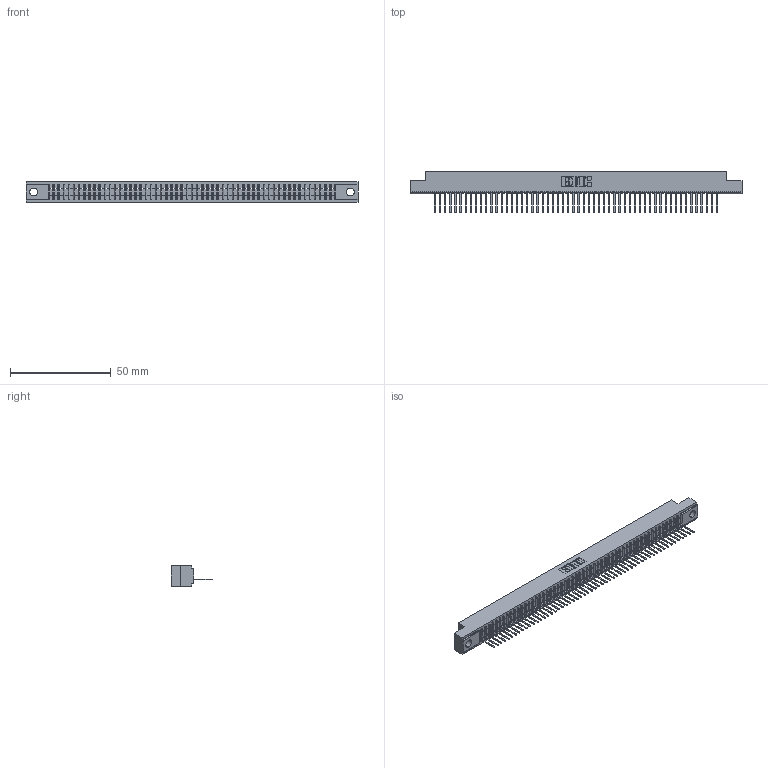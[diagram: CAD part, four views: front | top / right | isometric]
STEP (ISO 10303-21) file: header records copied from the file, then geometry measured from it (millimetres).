
FILE_DESCRIPTION (( 'STEP AP203' ), '1' );
FILE_NAME ('391-056-522-104.STEP', '2018-08-09T08:07:13', ( '' ), ( '' ), 'SwSTEP 2.0', 'SolidWorks 2016', '' );
FILE_SCHEMA (( 'CONFIG_CONTROL_DESIGN' ));
Length unit declared in the file: inch
Products named in the file (3): 341 Part_.156 (3.96) Dia Mounting Holes; 341-292-001_341-292-122; 391-056-522-104
Assembly tree (57 placements, depth 2):
  391-056-522-104
    341 Part_.156 (3.96) Dia Mounting Holes
    341-292-001_341-292-122  x56
Bounding box: 164.47 x 20.62 x 10.16 mm (x, y, z)
Volume: 11727.3 mm3; surface area: 18858.8 mm2
Topology: 57 solids, 57 shells, 4722 faces, 13624 edges, 8742 vertices
Faces by surface type: plane 2938, cylinder 1560, sphere 114, torus 110
Entity records: 64533 total; most frequent: CARTESIAN_POINT 10974, ORIENTED_EDGE 10960, DIRECTION 10574, EDGE_CURVE 5480, VECTOR 4450, LINE 4450, VERTEX_POINT 3462, AXIS2_PLACEMENT_3D 3062
